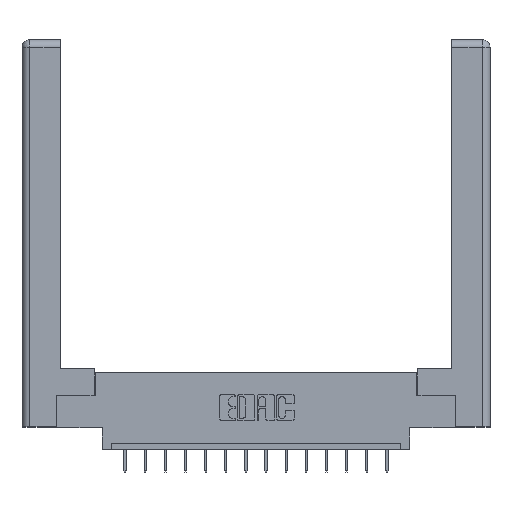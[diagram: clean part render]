
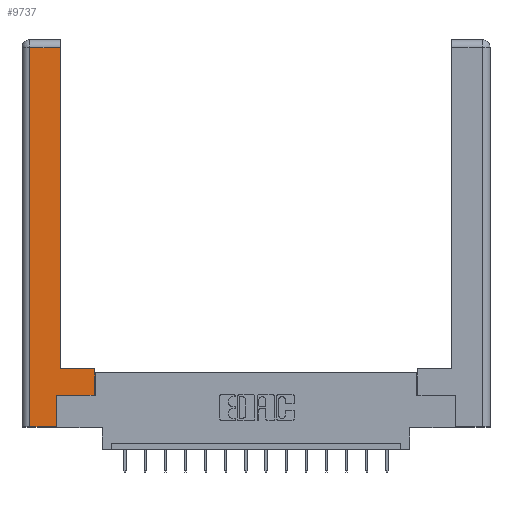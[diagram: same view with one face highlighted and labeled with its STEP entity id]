
A CAD part, top view. The second image highlights one B-rep face of the part: STEP entity #9737.
In plain terms, the highlighted planar face has unit normal (0, 0, 1).
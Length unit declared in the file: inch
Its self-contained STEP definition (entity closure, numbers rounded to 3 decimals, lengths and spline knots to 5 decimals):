
#66 = EDGE_CURVE ( 'NONE', #5365, #8915, #14595, .T. ) ;
#266 = EDGE_CURVE ( 'NONE', #3599, #16869, #5836, .T. ) ;
#676 = ORIENTED_EDGE ( 'NONE', *, *, #15440, .T. ) ;
#1061 = CARTESIAN_POINT ( 'NONE',  ( 0.0615, 2.94, 0. ) ) ;
#1191 = DIRECTION ( 'NONE',  ( -1., 0., 0. ) ) ;
#1420 = CARTESIAN_POINT ( 'NONE',  ( 0.265, 0., 0. ) ) ;
#1661 = DIRECTION ( 'NONE',  ( 0., 0., -1. ) ) ;
#1847 = CARTESIAN_POINT ( 'NONE',  ( 0.565, 0.45, 0. ) ) ;
#1917 = AXIS2_PLACEMENT_3D ( 'NONE', #13265, #1661, #16042 ) ;
#2126 = VECTOR ( 'NONE', #8145, 39.37008 ) ;
#2402 = CARTESIAN_POINT ( 'NONE',  ( 0.265, 0.245, 0. ) ) ;
#2893 = EDGE_CURVE ( 'NONE', #5746, #10574, #13285, .T. ) ;
#3107 = DIRECTION ( 'NONE',  ( 0., 1., 0. ) ) ;
#3453 = VECTOR ( 'NONE', #3107, 39.37008 ) ;
#3599 = VERTEX_POINT ( 'NONE', #2402 ) ;
#3629 = ORIENTED_EDGE ( 'NONE', *, *, #4790, .T. ) ;
#4346 = EDGE_CURVE ( 'NONE', #16869, #4712, #4647, .T. ) ;
#4580 = VECTOR ( 'NONE', #14454, 39.37008 ) ;
#4647 = LINE ( 'NONE', #1847, #16465 ) ;
#4712 = VERTEX_POINT ( 'NONE', #6523 ) ;
#4743 = LINE ( 'NONE', #11366, #15962 ) ;
#4790 = EDGE_CURVE ( 'NONE', #10574, #5365, #15856, .T. ) ;
#4793 = ORIENTED_EDGE ( 'NONE', *, *, #266, .T. ) ;
#5301 = CARTESIAN_POINT ( 'NONE',  ( 0.265, 0.245, 0. ) ) ;
#5365 = VERTEX_POINT ( 'NONE', #1061 ) ;
#5391 = CARTESIAN_POINT ( 'NONE',  ( 0.295, 0.45, 0. ) ) ;
#5746 = VERTEX_POINT ( 'NONE', #11276 ) ;
#5773 = CARTESIAN_POINT ( 'NONE',  ( 0.0615, 0., 0. ) ) ;
#5836 = LINE ( 'NONE', #13209, #4580 ) ;
#6005 = LINE ( 'NONE', #5301, #9043 ) ;
#6476 = DIRECTION ( 'NONE',  ( -1., 0., 0. ) ) ;
#6523 = CARTESIAN_POINT ( 'NONE',  ( 0.565, 0.45, 0. ) ) ;
#7095 = ORIENTED_EDGE ( 'NONE', *, *, #4346, .T. ) ;
#7158 = ORIENTED_EDGE ( 'NONE', *, *, #2893, .T. ) ;
#7330 = CARTESIAN_POINT ( 'NONE',  ( 0.565, 0.245, 0. ) ) ;
#7362 = EDGE_CURVE ( 'NONE', #12120, #3599, #6005, .T. ) ;
#7713 = CARTESIAN_POINT ( 'NONE',  ( 0.0615, 2.94, 0. ) ) ;
#8145 = DIRECTION ( 'NONE',  ( 0., -1., 0. ) ) ;
#8313 = CARTESIAN_POINT ( 'NONE',  ( 0.295, 3., 0. ) ) ;
#8659 = CARTESIAN_POINT ( 'NONE',  ( 0.295, 2.94, 0. ) ) ;
#8789 = FACE_OUTER_BOUND ( 'NONE', #12848, .T. ) ;
#8915 = VERTEX_POINT ( 'NONE', #13726 ) ;
#9010 = EDGE_CURVE ( 'NONE', #8915, #12120, #4743, .T. ) ;
#9041 = DIRECTION ( 'NONE',  ( 0., 1., 0. ) ) ;
#9043 = VECTOR ( 'NONE', #9041, 39.37008 ) ;
#9737 = ADVANCED_FACE ( 'NONE', ( #8789 ), #12172, .F. ) ;
#10574 = VERTEX_POINT ( 'NONE', #8659 ) ;
#11240 = ORIENTED_EDGE ( 'NONE', *, *, #7362, .T. ) ;
#11276 = CARTESIAN_POINT ( 'NONE',  ( 0.295, 0.45, 0. ) ) ;
#11366 = CARTESIAN_POINT ( 'NONE',  ( 0.265, 0., 0. ) ) ;
#12120 = VERTEX_POINT ( 'NONE', #1420 ) ;
#12172 = PLANE ( 'NONE',  #1917 ) ;
#12306 = VECTOR ( 'NONE', #6476, 39.37008 ) ;
#12403 = VECTOR ( 'NONE', #1191, 39.37008 ) ;
#12848 = EDGE_LOOP ( 'NONE', ( #7158, #3629, #13287, #15474, #11240, #4793, #7095, #676 ) ) ;
#13209 = CARTESIAN_POINT ( 'NONE',  ( 0.565, 0.245, 0. ) ) ;
#13265 = CARTESIAN_POINT ( 'NONE',  ( 0., 0., 0. ) ) ;
#13285 = LINE ( 'NONE', #8313, #3453 ) ;
#13287 = ORIENTED_EDGE ( 'NONE', *, *, #66, .T. ) ;
#13607 = DIRECTION ( 'NONE',  ( 0., 1., 0. ) ) ;
#13726 = CARTESIAN_POINT ( 'NONE',  ( 0.0615, 0., 0. ) ) ;
#14454 = DIRECTION ( 'NONE',  ( 1., 0., 0. ) ) ;
#14595 = LINE ( 'NONE', #5773, #2126 ) ;
#15087 = DIRECTION ( 'NONE',  ( 1., 0., 0. ) ) ;
#15440 = EDGE_CURVE ( 'NONE', #4712, #5746, #16770, .T. ) ;
#15474 = ORIENTED_EDGE ( 'NONE', *, *, #9010, .T. ) ;
#15856 = LINE ( 'NONE', #7713, #12403 ) ;
#15962 = VECTOR ( 'NONE', #15087, 39.37008 ) ;
#16042 = DIRECTION ( 'NONE',  ( -1., 0., 0. ) ) ;
#16465 = VECTOR ( 'NONE', #13607, 39.37008 ) ;
#16770 = LINE ( 'NONE', #5391, #12306 ) ;
#16869 = VERTEX_POINT ( 'NONE', #7330 ) ;
